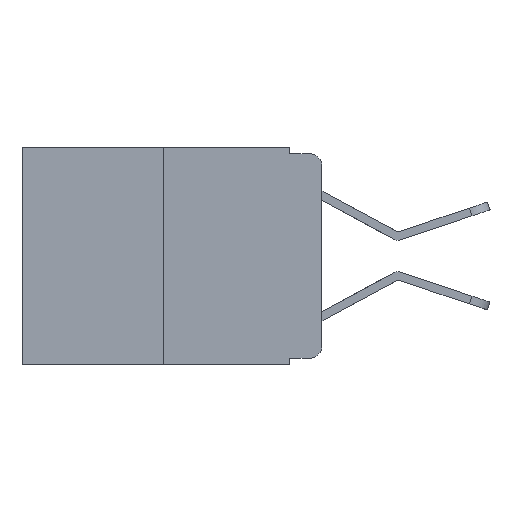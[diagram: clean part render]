
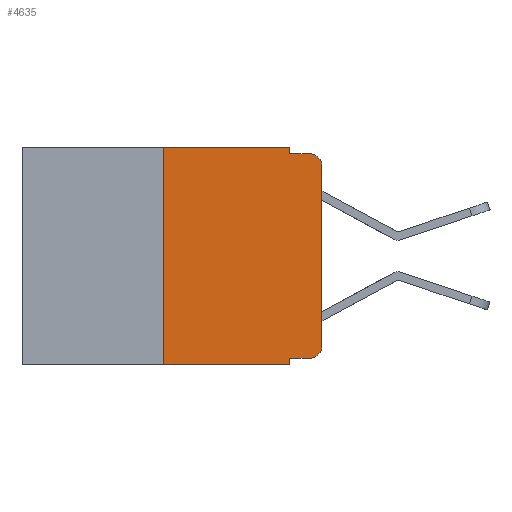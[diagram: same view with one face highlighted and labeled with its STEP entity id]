
A CAD part, left-side view. The second image highlights one B-rep face of the part: STEP entity #4635.
In plain terms, the highlighted planar face has unit normal (-1, 0, 0).
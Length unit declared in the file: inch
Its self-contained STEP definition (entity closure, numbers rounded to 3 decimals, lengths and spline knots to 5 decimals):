
#275 = AXIS2_PLACEMENT_3D ( 'NONE', #5809, #6028, #16174 ) ;
#360 = CARTESIAN_POINT ( 'NONE',  ( 0., 0.051, -0.333 ) ) ;
#369 = LINE ( 'NONE', #7081, #7911 ) ;
#994 = CARTESIAN_POINT ( 'NONE',  ( 0., 0.051, 0. ) ) ;
#1448 = ORIENTED_EDGE ( 'NONE', *, *, #10662, .F. ) ;
#1793 = CARTESIAN_POINT ( 'NONE',  ( 0., 0.051, 0. ) ) ;
#2109 = VERTEX_POINT ( 'NONE', #13249 ) ;
#2155 = DIRECTION ( 'NONE',  ( 0., 0., -1. ) ) ;
#2494 = DIRECTION ( 'NONE',  ( 0., 0., -1. ) ) ;
#2585 = ORIENTED_EDGE ( 'NONE', *, *, #10367, .F. ) ;
#3010 = CARTESIAN_POINT ( 'NONE',  ( 0., 0.051, 0. ) ) ;
#3255 = EDGE_LOOP ( 'NONE', ( #15091, #15928, #1448, #3363, #11678, #7128, #10948, #2585, #11516, #7282 ) ) ;
#3363 = ORIENTED_EDGE ( 'NONE', *, *, #5129, .F. ) ;
#4002 = VECTOR ( 'NONE', #2155, 39.37008 ) ;
#4248 = CARTESIAN_POINT ( 'NONE',  ( 0., 0.02, -0.333 ) ) ;
#4635 = ADVANCED_FACE ( 'NONE', ( #8094 ), #15764, .F. ) ;
#4832 = LINE ( 'NONE', #994, #4002 ) ;
#5129 = EDGE_CURVE ( 'NONE', #13313, #2109, #4832, .T. ) ;
#5250 = EDGE_CURVE ( 'NONE', #8193, #15421, #16004, .T. ) ;
#5809 = CARTESIAN_POINT ( 'NONE',  ( 0., 0.02, -0.313 ) ) ;
#5840 = VERTEX_POINT ( 'NONE', #11883 ) ;
#6028 = DIRECTION ( 'NONE',  ( -1., 0., 0. ) ) ;
#6068 = LINE ( 'NONE', #360, #9741 ) ;
#6107 = VECTOR ( 'NONE', #6150, 39.37008 ) ;
#6150 = DIRECTION ( 'NONE',  ( 0., 0., 1. ) ) ;
#6483 = CIRCLE ( 'NONE', #275, 0.02 ) ;
#6531 = DIRECTION ( 'NONE',  ( 0., 0., -1. ) ) ;
#6696 = VERTEX_POINT ( 'NONE', #13317 ) ;
#7020 = VERTEX_POINT ( 'NONE', #8562 ) ;
#7081 = CARTESIAN_POINT ( 'NONE',  ( 0., 0.473, 0. ) ) ;
#7128 = ORIENTED_EDGE ( 'NONE', *, *, #5250, .F. ) ;
#7282 = ORIENTED_EDGE ( 'NONE', *, *, #7501, .T. ) ;
#7501 = EDGE_CURVE ( 'NONE', #8397, #6696, #6483, .T. ) ;
#7614 = CARTESIAN_POINT ( 'NONE',  ( 0., 0.25, -0.343 ) ) ;
#7701 = CIRCLE ( 'NONE', #16754, 0.02 ) ;
#7831 = EDGE_CURVE ( 'NONE', #5840, #12583, #7701, .T. ) ;
#7911 = VECTOR ( 'NONE', #13702, 39.37008 ) ;
#8094 = FACE_OUTER_BOUND ( 'NONE', #3255, .T. ) ;
#8193 = VERTEX_POINT ( 'NONE', #7614 ) ;
#8397 = VERTEX_POINT ( 'NONE', #4248 ) ;
#8420 = DIRECTION ( 'NONE',  ( 0., 0., -1. ) ) ;
#8562 = CARTESIAN_POINT ( 'NONE',  ( 0., 0.051, -0.343 ) ) ;
#8677 = CARTESIAN_POINT ( 'NONE',  ( 0., 0.25, 0. ) ) ;
#8864 = DIRECTION ( 'NONE',  ( 0., -1., 0. ) ) ;
#9042 = DIRECTION ( 'NONE',  ( 0., 0., 1. ) ) ;
#9070 = CARTESIAN_POINT ( 'NONE',  ( 0., 0.473, -0.343 ) ) ;
#9487 = DIRECTION ( 'NONE',  ( 0., -1., 0. ) ) ;
#9741 = VECTOR ( 'NONE', #9487, 39.37008 ) ;
#10311 = DIRECTION ( 'NONE',  ( -1., 0., 0. ) ) ;
#10317 = VECTOR ( 'NONE', #9042, 39.37008 ) ;
#10367 = EDGE_CURVE ( 'NONE', #11398, #7020, #15966, .T. ) ;
#10459 = LINE ( 'NONE', #15467, #12517 ) ;
#10662 = EDGE_CURVE ( 'NONE', #2109, #12583, #10459, .T. ) ;
#10948 = ORIENTED_EDGE ( 'NONE', *, *, #11986, .T. ) ;
#11398 = VERTEX_POINT ( 'NONE', #11706 ) ;
#11516 = ORIENTED_EDGE ( 'NONE', *, *, #13280, .T. ) ;
#11678 = ORIENTED_EDGE ( 'NONE', *, *, #13436, .F. ) ;
#11706 = CARTESIAN_POINT ( 'NONE',  ( 0., 0.051, -0.333 ) ) ;
#11728 = AXIS2_PLACEMENT_3D ( 'NONE', #13110, #14467, #6531 ) ;
#11864 = EDGE_CURVE ( 'NONE', #6696, #5840, #16705, .T. ) ;
#11883 = CARTESIAN_POINT ( 'NONE',  ( 0., 0., -0.03 ) ) ;
#11986 = EDGE_CURVE ( 'NONE', #8193, #7020, #13065, .T. ) ;
#12517 = VECTOR ( 'NONE', #8864, 39.37008 ) ;
#12535 = VECTOR ( 'NONE', #8420, 39.37008 ) ;
#12583 = VERTEX_POINT ( 'NONE', #14204 ) ;
#12656 = VECTOR ( 'NONE', #14079, 39.37008 ) ;
#13065 = LINE ( 'NONE', #9070, #12656 ) ;
#13110 = CARTESIAN_POINT ( 'NONE',  ( 0., 0.473, 0. ) ) ;
#13249 = CARTESIAN_POINT ( 'NONE',  ( 0., 0.051, -0.01 ) ) ;
#13280 = EDGE_CURVE ( 'NONE', #11398, #8397, #6068, .T. ) ;
#13313 = VERTEX_POINT ( 'NONE', #1793 ) ;
#13317 = CARTESIAN_POINT ( 'NONE',  ( 0., 0., -0.313 ) ) ;
#13436 = EDGE_CURVE ( 'NONE', #15421, #13313, #369, .T. ) ;
#13702 = DIRECTION ( 'NONE',  ( 0., -1., 0. ) ) ;
#13964 = CARTESIAN_POINT ( 'NONE',  ( 0., 0., 0. ) ) ;
#14079 = DIRECTION ( 'NONE',  ( 0., -1., 0. ) ) ;
#14204 = CARTESIAN_POINT ( 'NONE',  ( 0., 0.02, -0.01 ) ) ;
#14467 = DIRECTION ( 'NONE',  ( 1., 0., 0. ) ) ;
#15091 = ORIENTED_EDGE ( 'NONE', *, *, #11864, .T. ) ;
#15421 = VERTEX_POINT ( 'NONE', #8677 ) ;
#15467 = CARTESIAN_POINT ( 'NONE',  ( 0., 0.051, -0.01 ) ) ;
#15517 = CARTESIAN_POINT ( 'NONE',  ( 0., 0.25, 0. ) ) ;
#15764 = PLANE ( 'NONE',  #11728 ) ;
#15928 = ORIENTED_EDGE ( 'NONE', *, *, #7831, .T. ) ;
#15966 = LINE ( 'NONE', #3010, #12535 ) ;
#16004 = LINE ( 'NONE', #15517, #10317 ) ;
#16174 = DIRECTION ( 'NONE',  ( 0., 0., -1. ) ) ;
#16705 = LINE ( 'NONE', #13964, #6107 ) ;
#16754 = AXIS2_PLACEMENT_3D ( 'NONE', #16774, #10311, #2494 ) ;
#16774 = CARTESIAN_POINT ( 'NONE',  ( 0., 0.02, -0.03 ) ) ;
